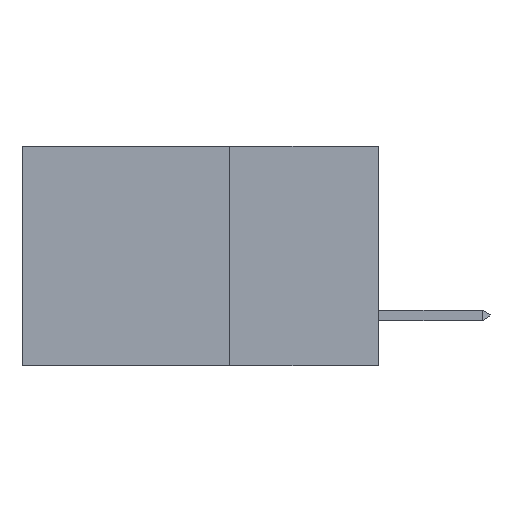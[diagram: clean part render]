
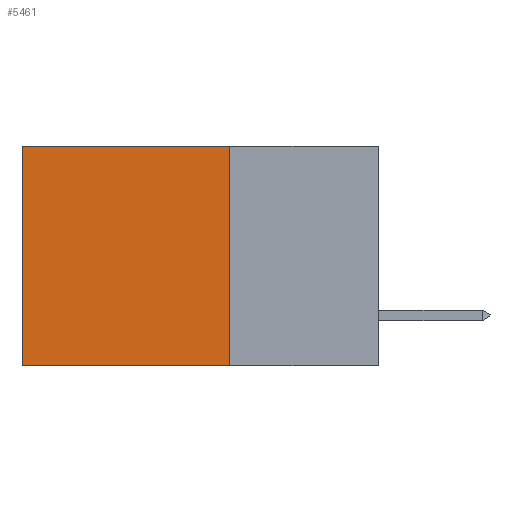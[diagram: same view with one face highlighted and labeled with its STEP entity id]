
A CAD part, left-side view. The second image highlights one B-rep face of the part: STEP entity #5461.
In plain terms, the highlighted planar face has unit normal (-1, 0, 0).
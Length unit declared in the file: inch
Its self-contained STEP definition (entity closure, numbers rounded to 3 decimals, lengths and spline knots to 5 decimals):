
#274 = LINE ( 'NONE', #2349, #4671 ) ;
#654 = LINE ( 'NONE', #1541, #2095 ) ;
#1053 = CARTESIAN_POINT ( 'NONE',  ( 0.2615, 0.25, -0.37 ) ) ;
#1097 = DIRECTION ( 'NONE',  ( 0., 1., 0. ) ) ;
#1148 = CARTESIAN_POINT ( 'NONE',  ( 0.2615, 0.25, -0.37 ) ) ;
#1364 = VERTEX_POINT ( 'NONE', #2399 ) ;
#1416 = CARTESIAN_POINT ( 'NONE',  ( 0.2615, 0.25, -0.37 ) ) ;
#1422 = VERTEX_POINT ( 'NONE', #4052 ) ;
#1541 = CARTESIAN_POINT ( 'NONE',  ( 0.2615, 0.25, 0. ) ) ;
#1879 = EDGE_CURVE ( 'NONE', #1422, #4481, #5489, .T. ) ;
#2095 = VECTOR ( 'NONE', #8028, 39.37008 ) ;
#2163 = CARTESIAN_POINT ( 'NONE',  ( 0.2615, 0.6, 0. ) ) ;
#2349 = CARTESIAN_POINT ( 'NONE',  ( 0.2615, 0.6, -0.37 ) ) ;
#2399 = CARTESIAN_POINT ( 'NONE',  ( 0.2615, 0.25, 0. ) ) ;
#2621 = EDGE_LOOP ( 'NONE', ( #4962, #5431, #5502, #4759 ) ) ;
#2699 = VECTOR ( 'NONE', #1097, 39.37008 ) ;
#3138 = CARTESIAN_POINT ( 'NONE',  ( 0.2615, 0.6, -0.37 ) ) ;
#3964 = DIRECTION ( 'NONE',  ( 1., 0., 0. ) ) ;
#4003 = PLANE ( 'NONE',  #6896 ) ;
#4052 = CARTESIAN_POINT ( 'NONE',  ( 0.2615, 0.25, -0.37 ) ) ;
#4481 = VERTEX_POINT ( 'NONE', #3138 ) ;
#4530 = DIRECTION ( 'NONE',  ( 0., 0., -1. ) ) ;
#4671 = VECTOR ( 'NONE', #4530, 39.37008 ) ;
#4759 = ORIENTED_EDGE ( 'NONE', *, *, #7459, .T. ) ;
#4771 = DIRECTION ( 'NONE',  ( 0., 0., -1. ) ) ;
#4962 = ORIENTED_EDGE ( 'NONE', *, *, #9146, .T. ) ;
#5086 = VERTEX_POINT ( 'NONE', #2163 ) ;
#5412 = VECTOR ( 'NONE', #7164, 39.37008 ) ;
#5431 = ORIENTED_EDGE ( 'NONE', *, *, #1879, .F. ) ;
#5461 = ADVANCED_FACE ( 'NONE', ( #7584 ), #4003, .F. ) ;
#5489 = LINE ( 'NONE', #1148, #2699 ) ;
#5502 = ORIENTED_EDGE ( 'NONE', *, *, #6503, .F. ) ;
#6503 = EDGE_CURVE ( 'NONE', #1364, #1422, #7853, .T. ) ;
#6896 = AXIS2_PLACEMENT_3D ( 'NONE', #1053, #3964, #4771 ) ;
#7164 = DIRECTION ( 'NONE',  ( 0., 0., -1. ) ) ;
#7459 = EDGE_CURVE ( 'NONE', #1364, #5086, #654, .T. ) ;
#7584 = FACE_OUTER_BOUND ( 'NONE', #2621, .T. ) ;
#7853 = LINE ( 'NONE', #1416, #5412 ) ;
#8028 = DIRECTION ( 'NONE',  ( 0., 1., 0. ) ) ;
#9146 = EDGE_CURVE ( 'NONE', #5086, #4481, #274, .T. ) ;
